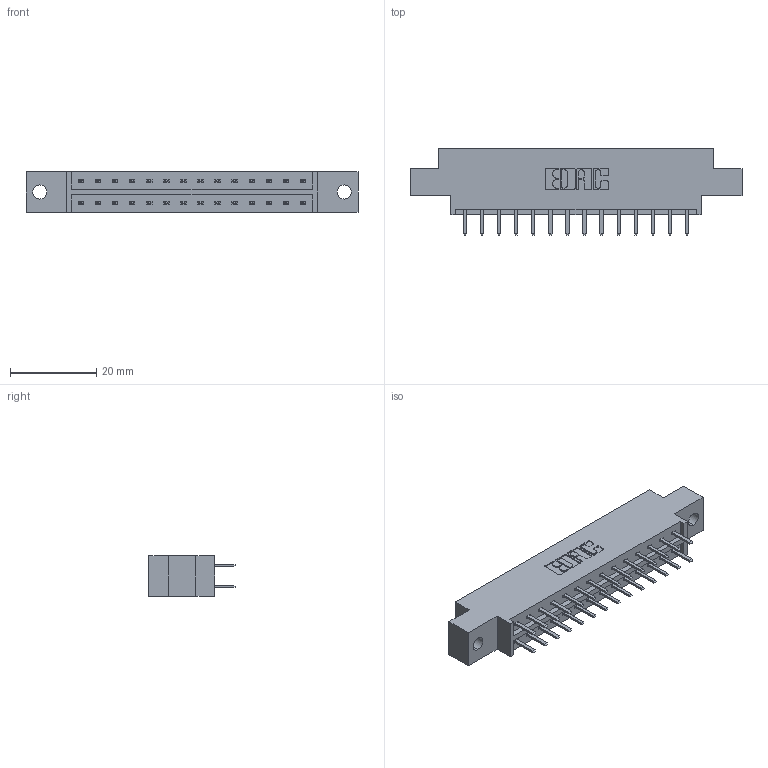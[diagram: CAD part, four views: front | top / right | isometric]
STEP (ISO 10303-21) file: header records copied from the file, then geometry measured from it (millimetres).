
FILE_DESCRIPTION (( 'STEP AP203' ), '1' );
FILE_NAME ('833-028-520-802.STEP', '2020-06-02T07:46:07', ( '' ), ( '' ), 'SwSTEP 2.0', 'SolidWorks 2020', '' );
FILE_SCHEMA (( 'CONFIG_CONTROL_DESIGN' ));
Length unit declared in the file: inch
Products named in the file (3): 833-028-520-802; 345-292-001_345-293-120; 833 Part_Offset - .128 Dia
Assembly tree (29 placements, depth 2):
  833-028-520-802
    833 Part_Offset - .128 Dia
    345-292-001_345-293-120  x28
Bounding box: 77.01 x 20.02 x 9.4 mm (x, y, z)
Volume: 7323.9 mm3; surface area: 8272.7 mm2
Topology: 29 solids, 29 shells, 1686 faces, 4887 edges, 3182 vertices
Faces by surface type: plane 1138, cylinder 548
Entity records: 12877 total; most frequent: CARTESIAN_POINT 2182, ORIENTED_EDGE 2106, DIRECTION 1901, EDGE_CURVE 1053, LINE 921, VECTOR 921, VERTEX_POINT 698, AXIS2_PLACEMENT_3D 490
